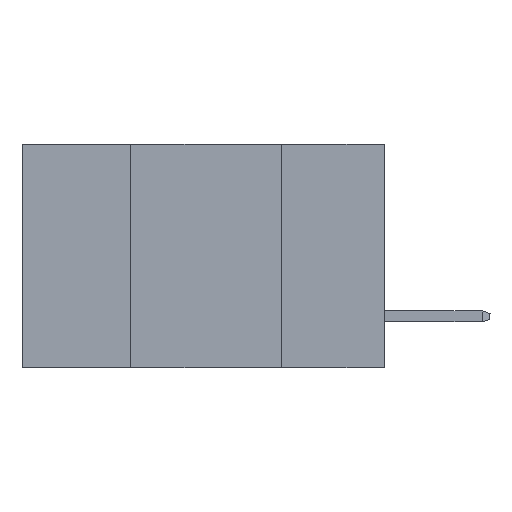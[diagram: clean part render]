
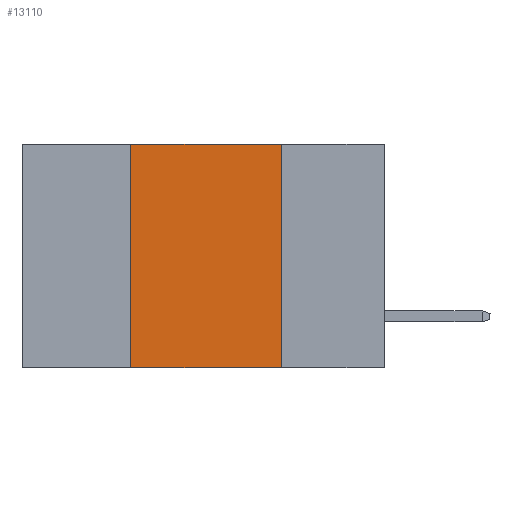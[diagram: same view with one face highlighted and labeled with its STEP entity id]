
A CAD part, left-side view. The second image highlights one B-rep face of the part: STEP entity #13110.
In plain terms, the highlighted planar face has unit normal (-1, 0, 0).
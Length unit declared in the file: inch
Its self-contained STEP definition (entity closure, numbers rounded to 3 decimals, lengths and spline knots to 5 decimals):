
#335 = EDGE_LOOP ( 'NONE', ( #2911, #5002, #23253, #23829 ) ) ;
#945 = CARTESIAN_POINT ( 'NONE',  ( 0., 0.6, 0. ) ) ;
#1322 = DIRECTION ( 'NONE',  ( 0., 0., -1. ) ) ;
#2887 = DIRECTION ( 'NONE',  ( 1., 0., 0. ) ) ;
#2911 = ORIENTED_EDGE ( 'NONE', *, *, #23937, .F. ) ;
#2955 = EDGE_CURVE ( 'NONE', #10432, #3941, #14810, .T. ) ;
#3562 = VECTOR ( 'NONE', #6016, 39.37008 ) ;
#3941 = VERTEX_POINT ( 'NONE', #12495 ) ;
#3952 = LINE ( 'NONE', #17587, #3562 ) ;
#5002 = ORIENTED_EDGE ( 'NONE', *, *, #2955, .F. ) ;
#5923 = DIRECTION ( 'NONE',  ( 0., -1., 0. ) ) ;
#6016 = DIRECTION ( 'NONE',  ( 0., 0., -1. ) ) ;
#6164 = VECTOR ( 'NONE', #24573, 39.37008 ) ;
#7373 = CARTESIAN_POINT ( 'NONE',  ( 0., 0.42, -0.37 ) ) ;
#9203 = FACE_OUTER_BOUND ( 'NONE', #335, .T. ) ;
#9879 = VERTEX_POINT ( 'NONE', #13466 ) ;
#9908 = CARTESIAN_POINT ( 'NONE',  ( 0., 0.6, -0.37 ) ) ;
#10278 = AXIS2_PLACEMENT_3D ( 'NONE', #945, #2887, #1322 ) ;
#10432 = VERTEX_POINT ( 'NONE', #12144 ) ;
#10823 = VECTOR ( 'NONE', #5923, 39.37008 ) ;
#10831 = CARTESIAN_POINT ( 'NONE',  ( 0., 0.6, 0. ) ) ;
#11534 = EDGE_CURVE ( 'NONE', #20532, #10432, #13700, .T. ) ;
#12144 = CARTESIAN_POINT ( 'NONE',  ( 0., 0.42, 0. ) ) ;
#12495 = CARTESIAN_POINT ( 'NONE',  ( 0., 0.17, 0. ) ) ;
#13110 = ADVANCED_FACE ( 'NONE', ( #9203 ), #24358, .F. ) ;
#13466 = CARTESIAN_POINT ( 'NONE',  ( 0., 0.17, -0.37 ) ) ;
#13700 = LINE ( 'NONE', #25275, #17080 ) ;
#14810 = LINE ( 'NONE', #10831, #6164 ) ;
#15680 = LINE ( 'NONE', #9908, #10823 ) ;
#17080 = VECTOR ( 'NONE', #21402, 39.37008 ) ;
#17587 = CARTESIAN_POINT ( 'NONE',  ( 0., 0.17, -0.37 ) ) ;
#18520 = EDGE_CURVE ( 'NONE', #20532, #9879, #15680, .T. ) ;
#20532 = VERTEX_POINT ( 'NONE', #7373 ) ;
#21402 = DIRECTION ( 'NONE',  ( 0., 0., 1. ) ) ;
#23253 = ORIENTED_EDGE ( 'NONE', *, *, #11534, .F. ) ;
#23829 = ORIENTED_EDGE ( 'NONE', *, *, #18520, .T. ) ;
#23937 = EDGE_CURVE ( 'NONE', #3941, #9879, #3952, .T. ) ;
#24358 = PLANE ( 'NONE',  #10278 ) ;
#24573 = DIRECTION ( 'NONE',  ( 0., -1., 0. ) ) ;
#25275 = CARTESIAN_POINT ( 'NONE',  ( 0., 0.42, -0.37 ) ) ;
